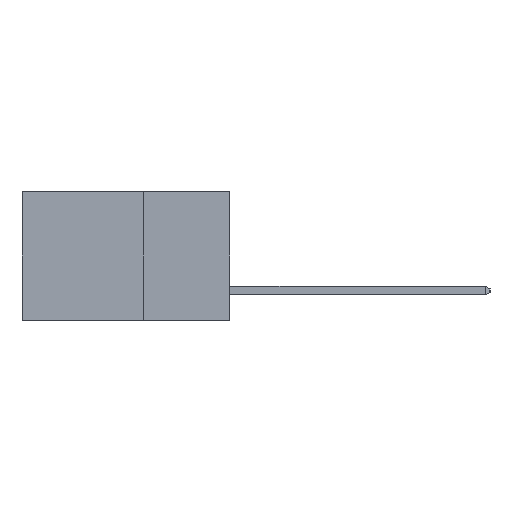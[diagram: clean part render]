
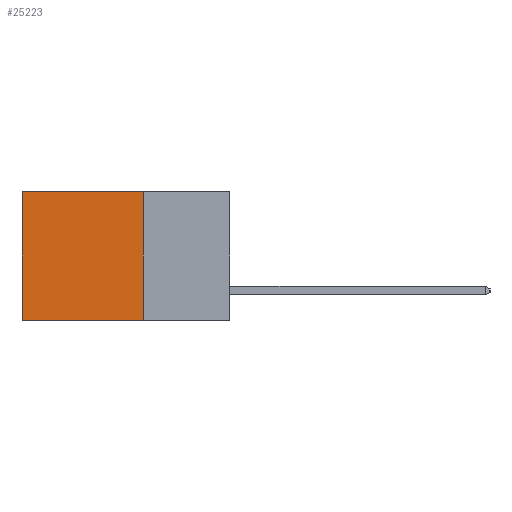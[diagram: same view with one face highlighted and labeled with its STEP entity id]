
A CAD part, left-side view. The second image highlights one B-rep face of the part: STEP entity #25223.
In plain terms, the highlighted planar face has unit normal (-1, 0, 0).
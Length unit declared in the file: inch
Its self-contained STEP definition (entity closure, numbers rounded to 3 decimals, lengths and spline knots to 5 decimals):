
#831 = VERTEX_POINT ( 'NONE', #5130 ) ;
#952 = ORIENTED_EDGE ( 'NONE', *, *, #8532, .T. ) ;
#1086 = DIRECTION ( 'NONE',  ( 0., 0., -1. ) ) ;
#1126 = VERTEX_POINT ( 'NONE', #3490 ) ;
#1533 = VECTOR ( 'NONE', #1086, 39.37008 ) ;
#2173 = EDGE_LOOP ( 'NONE', ( #952, #19389, #2919, #11501 ) ) ;
#2583 = VECTOR ( 'NONE', #12918, 39.37008 ) ;
#2810 = VECTOR ( 'NONE', #17975, 39.37008 ) ;
#2919 = ORIENTED_EDGE ( 'NONE', *, *, #6911, .F. ) ;
#3490 = CARTESIAN_POINT ( 'NONE',  ( 0.298, 0.25, 0. ) ) ;
#5130 = CARTESIAN_POINT ( 'NONE',  ( 0.298, 0.6, -0.37 ) ) ;
#6139 = VERTEX_POINT ( 'NONE', #10645 ) ;
#6911 = EDGE_CURVE ( 'NONE', #1126, #21893, #7558, .T. ) ;
#6947 = DIRECTION ( 'NONE',  ( 0., 0., -1. ) ) ;
#7558 = LINE ( 'NONE', #21009, #1533 ) ;
#8342 = CARTESIAN_POINT ( 'NONE',  ( 0.298, 0.25, -0.37 ) ) ;
#8532 = EDGE_CURVE ( 'NONE', #6139, #831, #18504, .T. ) ;
#8859 = PLANE ( 'NONE',  #12203 ) ;
#8971 = CARTESIAN_POINT ( 'NONE',  ( 0.298, 0.25, 0. ) ) ;
#10645 = CARTESIAN_POINT ( 'NONE',  ( 0.298, 0.6, 0. ) ) ;
#11041 = FACE_OUTER_BOUND ( 'NONE', #2173, .T. ) ;
#11501 = ORIENTED_EDGE ( 'NONE', *, *, #17503, .T. ) ;
#12203 = AXIS2_PLACEMENT_3D ( 'NONE', #12821, #18623, #6947 ) ;
#12821 = CARTESIAN_POINT ( 'NONE',  ( 0.298, 0.25, 0. ) ) ;
#12918 = DIRECTION ( 'NONE',  ( 0., 1., 0. ) ) ;
#13066 = CARTESIAN_POINT ( 'NONE',  ( 0.298, 0.25, -0.37 ) ) ;
#13173 = LINE ( 'NONE', #8971, #2583 ) ;
#13648 = VECTOR ( 'NONE', #16223, 39.37008 ) ;
#16070 = CARTESIAN_POINT ( 'NONE',  ( 0.298, 0.6, 0. ) ) ;
#16223 = DIRECTION ( 'NONE',  ( 0., 1., 0. ) ) ;
#17503 = EDGE_CURVE ( 'NONE', #1126, #6139, #13173, .T. ) ;
#17975 = DIRECTION ( 'NONE',  ( 0., 0., -1. ) ) ;
#18504 = LINE ( 'NONE', #16070, #2810 ) ;
#18623 = DIRECTION ( 'NONE',  ( 1., 0., 0. ) ) ;
#18798 = LINE ( 'NONE', #8342, #13648 ) ;
#19212 = EDGE_CURVE ( 'NONE', #21893, #831, #18798, .T. ) ;
#19389 = ORIENTED_EDGE ( 'NONE', *, *, #19212, .F. ) ;
#21009 = CARTESIAN_POINT ( 'NONE',  ( 0.298, 0.25, 0. ) ) ;
#21893 = VERTEX_POINT ( 'NONE', #13066 ) ;
#25223 = ADVANCED_FACE ( 'NONE', ( #11041 ), #8859, .F. ) ;
